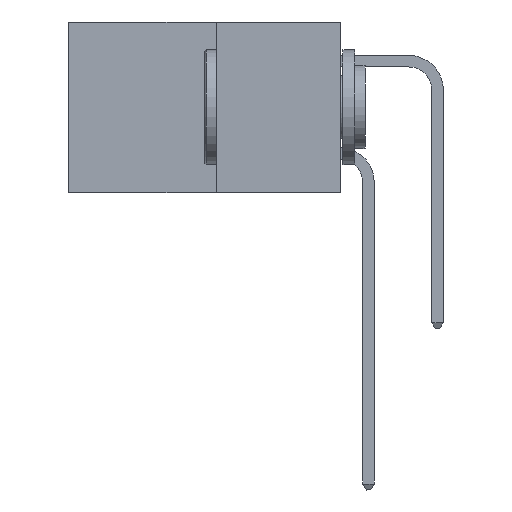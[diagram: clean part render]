
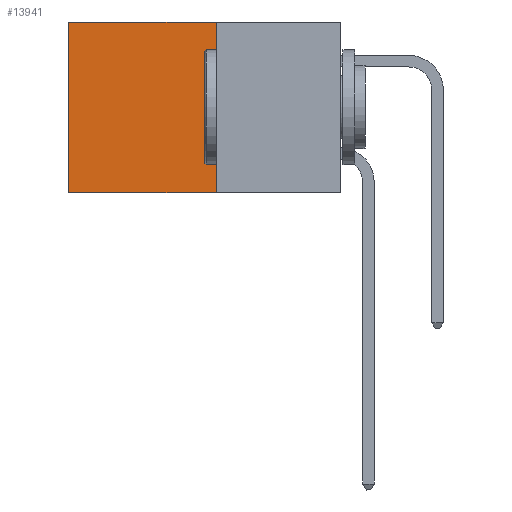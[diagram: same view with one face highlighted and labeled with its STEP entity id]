
A CAD part, left-side view. The second image highlights one B-rep face of the part: STEP entity #13941.
In plain terms, the highlighted planar face has unit normal (-1, 0, 0).
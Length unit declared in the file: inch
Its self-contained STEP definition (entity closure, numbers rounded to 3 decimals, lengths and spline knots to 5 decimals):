
#39 = VECTOR ( 'NONE', #119, 39.37008 ) ;
#119 = DIRECTION ( 'NONE',  ( 0., 1., 0. ) ) ;
#462 = EDGE_CURVE ( 'NONE', #17707, #1313, #3896, .T. ) ;
#1313 = VERTEX_POINT ( 'NONE', #9888 ) ;
#2470 = CARTESIAN_POINT ( 'NONE',  ( 0.277, 0.27, -0.37 ) ) ;
#3461 = VECTOR ( 'NONE', #4348, 39.37008 ) ;
#3690 = ORIENTED_EDGE ( 'NONE', *, *, #18618, .T. ) ;
#3896 = LINE ( 'NONE', #6130, #12351 ) ;
#4348 = DIRECTION ( 'NONE',  ( 0., 0., -1. ) ) ;
#5717 = DIRECTION ( 'NONE',  ( 0., 1., 0. ) ) ;
#6130 = CARTESIAN_POINT ( 'NONE',  ( 0.277, 0.27, -0.37 ) ) ;
#6416 = VERTEX_POINT ( 'NONE', #19111 ) ;
#7153 = AXIS2_PLACEMENT_3D ( 'NONE', #18086, #8185, #19720 ) ;
#8069 = LINE ( 'NONE', #9416, #3461 ) ;
#8075 = LINE ( 'NONE', #15474, #16407 ) ;
#8185 = DIRECTION ( 'NONE',  ( 1., 0., 0. ) ) ;
#8886 = ORIENTED_EDGE ( 'NONE', *, *, #14225, .F. ) ;
#9188 = LINE ( 'NONE', #10360, #39 ) ;
#9416 = CARTESIAN_POINT ( 'NONE',  ( 0.277, 0.59, -0.37 ) ) ;
#9888 = CARTESIAN_POINT ( 'NONE',  ( 0.277, 0.59, -0.37 ) ) ;
#10324 = VERTEX_POINT ( 'NONE', #16594 ) ;
#10360 = CARTESIAN_POINT ( 'NONE',  ( 0.277, 0.27, 0. ) ) ;
#11326 = ORIENTED_EDGE ( 'NONE', *, *, #462, .F. ) ;
#12209 = FACE_OUTER_BOUND ( 'NONE', #16114, .T. ) ;
#12351 = VECTOR ( 'NONE', #5717, 39.37008 ) ;
#13941 = ADVANCED_FACE ( 'NONE', ( #12209 ), #19652, .F. ) ;
#14225 = EDGE_CURVE ( 'NONE', #10324, #17707, #8075, .T. ) ;
#15474 = CARTESIAN_POINT ( 'NONE',  ( 0.277, 0.27, -0.37 ) ) ;
#15779 = ORIENTED_EDGE ( 'NONE', *, *, #19487, .T. ) ;
#16114 = EDGE_LOOP ( 'NONE', ( #15779, #11326, #8886, #3690 ) ) ;
#16407 = VECTOR ( 'NONE', #17119, 39.37008 ) ;
#16594 = CARTESIAN_POINT ( 'NONE',  ( 0.277, 0.27, 0. ) ) ;
#17119 = DIRECTION ( 'NONE',  ( 0., 0., -1. ) ) ;
#17707 = VERTEX_POINT ( 'NONE', #2470 ) ;
#18086 = CARTESIAN_POINT ( 'NONE',  ( 0.277, 0.27, -0.37 ) ) ;
#18618 = EDGE_CURVE ( 'NONE', #10324, #6416, #9188, .T. ) ;
#19111 = CARTESIAN_POINT ( 'NONE',  ( 0.277, 0.59, 0. ) ) ;
#19487 = EDGE_CURVE ( 'NONE', #6416, #1313, #8069, .T. ) ;
#19652 = PLANE ( 'NONE',  #7153 ) ;
#19720 = DIRECTION ( 'NONE',  ( 0., 0., -1. ) ) ;
